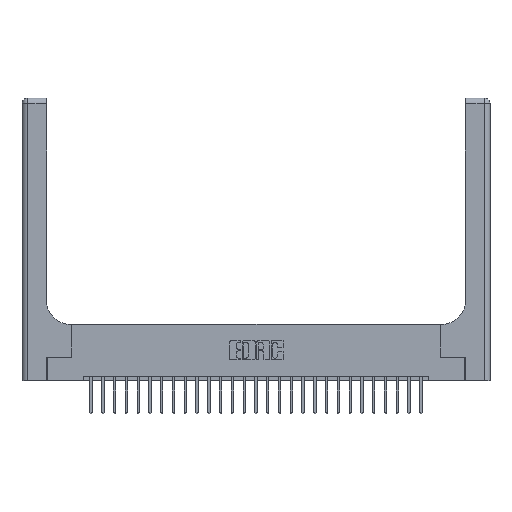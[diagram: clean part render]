
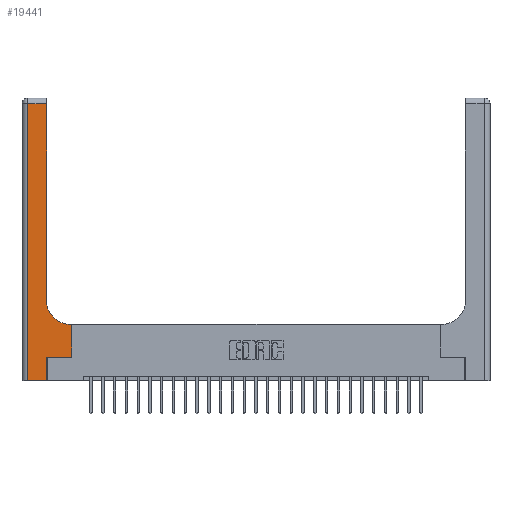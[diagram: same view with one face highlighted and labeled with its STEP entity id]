
A CAD part, top view. The second image highlights one B-rep face of the part: STEP entity #19441.
In plain terms, the highlighted planar face has unit normal (0, 0, 1).
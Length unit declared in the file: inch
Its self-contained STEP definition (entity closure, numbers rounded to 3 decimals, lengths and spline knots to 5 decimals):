
#158 = LINE ( 'NONE', #1902, #1753 ) ;
#548 = DIRECTION ( 'NONE',  ( 0., 0., -1. ) ) ;
#681 = EDGE_CURVE ( 'NONE', #15326, #17405, #17466, .T. ) ;
#783 = DIRECTION ( 'NONE',  ( 0., 1., 0. ) ) ;
#1055 = CARTESIAN_POINT ( 'NONE',  ( 0.528, 0.6, 0.37 ) ) ;
#1649 = VERTEX_POINT ( 'NONE', #10397 ) ;
#1753 = VECTOR ( 'NONE', #14291, 39.37008 ) ;
#1902 = CARTESIAN_POINT ( 'NONE',  ( 0., 0., 0.37 ) ) ;
#2203 = ORIENTED_EDGE ( 'NONE', *, *, #3390, .T. ) ;
#2357 = DIRECTION ( 'NONE',  ( 0., -1., 0. ) ) ;
#2428 = EDGE_CURVE ( 'NONE', #19091, #15475, #10344, .T. ) ;
#2664 = FACE_OUTER_BOUND ( 'NONE', #5003, .T. ) ;
#2775 = LINE ( 'NONE', #19045, #13738 ) ;
#2858 = DIRECTION ( 'NONE',  ( 0., 1., 0. ) ) ;
#2957 = EDGE_CURVE ( 'NONE', #1649, #19091, #7889, .T. ) ;
#3051 = ORIENTED_EDGE ( 'NONE', *, *, #19472, .T. ) ;
#3059 = CARTESIAN_POINT ( 'NONE',  ( 0., 3., 0.37 ) ) ;
#3171 = ORIENTED_EDGE ( 'NONE', *, *, #681, .T. ) ;
#3185 = DIRECTION ( 'NONE',  ( 1., 0., 0. ) ) ;
#3262 = AXIS2_PLACEMENT_3D ( 'NONE', #3059, #548, #21175 ) ;
#3390 = EDGE_CURVE ( 'NONE', #15475, #22272, #158, .T. ) ;
#3792 = DIRECTION ( 'NONE',  ( 0., 1., 0. ) ) ;
#4036 = DIRECTION ( 'NONE',  ( -1., 0., 0. ) ) ;
#5003 = EDGE_LOOP ( 'NONE', ( #14600, #15267, #17541, #2203, #6616, #3051, #9303, #19087, #3171 ) ) ;
#5187 = EDGE_CURVE ( 'NONE', #17405, #1649, #2775, .T. ) ;
#5305 = CARTESIAN_POINT ( 'NONE',  ( 0.265, 0., 0.37 ) ) ;
#5667 = LINE ( 'NONE', #13806, #25483 ) ;
#5912 = AXIS2_PLACEMENT_3D ( 'NONE', #15134, #22866, #17292 ) ;
#6151 = CARTESIAN_POINT ( 'NONE',  ( 0.26, 0.6, 0.37 ) ) ;
#6616 = ORIENTED_EDGE ( 'NONE', *, *, #12108, .T. ) ;
#7709 = VECTOR ( 'NONE', #4036, 39.37008 ) ;
#7889 = LINE ( 'NONE', #18477, #7709 ) ;
#8832 = CARTESIAN_POINT ( 'NONE',  ( 0.265, 0., 0.37 ) ) ;
#9303 = ORIENTED_EDGE ( 'NONE', *, *, #21449, .T. ) ;
#10344 = LINE ( 'NONE', #16513, #20047 ) ;
#10397 = CARTESIAN_POINT ( 'NONE',  ( 0.26, 2.94, 0.37 ) ) ;
#10918 = CARTESIAN_POINT ( 'NONE',  ( 0.265, 0.25, 0.37 ) ) ;
#11341 = CARTESIAN_POINT ( 'NONE',  ( 0.06, 2.94, 0.37 ) ) ;
#12108 = EDGE_CURVE ( 'NONE', #22272, #26171, #12979, .T. ) ;
#12310 = VERTEX_POINT ( 'NONE', #23914 ) ;
#12979 = LINE ( 'NONE', #8832, #22994 ) ;
#13171 = PLANE ( 'NONE',  #3262 ) ;
#13555 = VERTEX_POINT ( 'NONE', #1055 ) ;
#13738 = VECTOR ( 'NONE', #783, 39.37008 ) ;
#13806 = CARTESIAN_POINT ( 'NONE',  ( 0.528, 0.25, 0.37 ) ) ;
#14251 = CARTESIAN_POINT ( 'NONE',  ( 0.51, 0.6, 0.37 ) ) ;
#14291 = DIRECTION ( 'NONE',  ( 1., 0., 0. ) ) ;
#14600 = ORIENTED_EDGE ( 'NONE', *, *, #5187, .T. ) ;
#15134 = CARTESIAN_POINT ( 'NONE',  ( 0.51, 0.85, 0.37 ) ) ;
#15267 = ORIENTED_EDGE ( 'NONE', *, *, #2957, .T. ) ;
#15326 = VERTEX_POINT ( 'NONE', #14251 ) ;
#15475 = VERTEX_POINT ( 'NONE', #24786 ) ;
#16331 = LINE ( 'NONE', #6151, #20000 ) ;
#16513 = CARTESIAN_POINT ( 'NONE',  ( 0.06, 3., 0.37 ) ) ;
#17292 = DIRECTION ( 'NONE',  ( 1., 0., 0. ) ) ;
#17405 = VERTEX_POINT ( 'NONE', #17694 ) ;
#17466 = CIRCLE ( 'NONE', #5912, 0.25 ) ;
#17541 = ORIENTED_EDGE ( 'NONE', *, *, #2428, .T. ) ;
#17694 = CARTESIAN_POINT ( 'NONE',  ( 0.26, 0.85, 0.37 ) ) ;
#18477 = CARTESIAN_POINT ( 'NONE',  ( 0., 2.94, 0.37 ) ) ;
#19045 = CARTESIAN_POINT ( 'NONE',  ( 0.26, 3., 0.37 ) ) ;
#19087 = ORIENTED_EDGE ( 'NONE', *, *, #24808, .T. ) ;
#19091 = VERTEX_POINT ( 'NONE', #11341 ) ;
#19331 = LINE ( 'NONE', #10918, #21593 ) ;
#19441 = ADVANCED_FACE ( 'NONE', ( #2664 ), #13171, .F. ) ;
#19472 = EDGE_CURVE ( 'NONE', #26171, #12310, #19331, .T. ) ;
#20000 = VECTOR ( 'NONE', #24444, 39.37008 ) ;
#20047 = VECTOR ( 'NONE', #2357, 39.37008 ) ;
#20960 = CARTESIAN_POINT ( 'NONE',  ( 0.265, 0.25, 0.37 ) ) ;
#21175 = DIRECTION ( 'NONE',  ( -1., 0., 0. ) ) ;
#21449 = EDGE_CURVE ( 'NONE', #12310, #13555, #5667, .T. ) ;
#21593 = VECTOR ( 'NONE', #3185, 39.37008 ) ;
#22272 = VERTEX_POINT ( 'NONE', #5305 ) ;
#22866 = DIRECTION ( 'NONE',  ( 0., 0., -1. ) ) ;
#22994 = VECTOR ( 'NONE', #2858, 39.37008 ) ;
#23914 = CARTESIAN_POINT ( 'NONE',  ( 0.528, 0.25, 0.37 ) ) ;
#24444 = DIRECTION ( 'NONE',  ( -1., 0., 0. ) ) ;
#24786 = CARTESIAN_POINT ( 'NONE',  ( 0.06, 0., 0.37 ) ) ;
#24808 = EDGE_CURVE ( 'NONE', #13555, #15326, #16331, .T. ) ;
#25483 = VECTOR ( 'NONE', #3792, 39.37008 ) ;
#26171 = VERTEX_POINT ( 'NONE', #20960 ) ;
